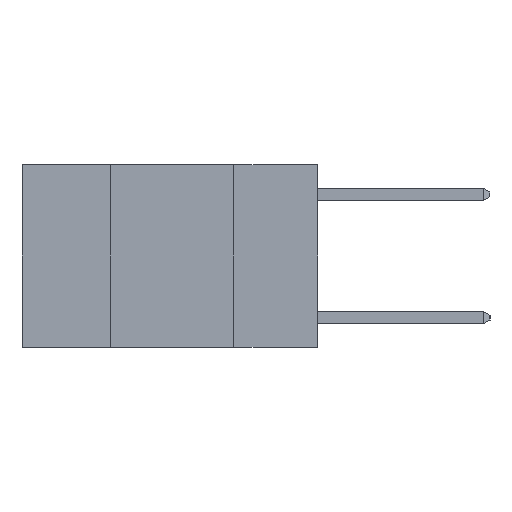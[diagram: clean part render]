
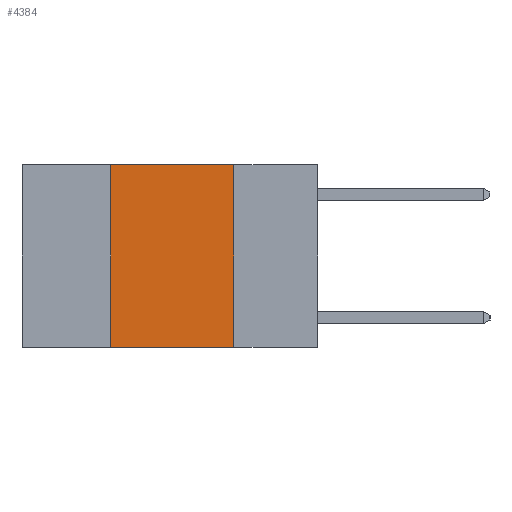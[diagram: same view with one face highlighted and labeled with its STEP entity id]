
A CAD part, left-side view. The second image highlights one B-rep face of the part: STEP entity #4384.
In plain terms, the highlighted planar face has unit normal (-1, 0, 0).
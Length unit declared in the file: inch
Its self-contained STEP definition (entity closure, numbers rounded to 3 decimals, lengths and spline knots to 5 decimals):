
#408 = CARTESIAN_POINT ( 'NONE',  ( 0., 0.17, 0. ) ) ;
#870 = FACE_OUTER_BOUND ( 'NONE', #2531, .T. ) ;
#1469 = CARTESIAN_POINT ( 'NONE',  ( 0., 0.42, -0.37 ) ) ;
#1685 = VERTEX_POINT ( 'NONE', #2592 ) ;
#1968 = VERTEX_POINT ( 'NONE', #1469 ) ;
#2078 = CARTESIAN_POINT ( 'NONE',  ( 0., 0.17, 0. ) ) ;
#2221 = VECTOR ( 'NONE', #9782, 39.37008 ) ;
#2294 = VECTOR ( 'NONE', #6770, 39.37008 ) ;
#2531 = EDGE_LOOP ( 'NONE', ( #7770, #8087, #8686, #8904 ) ) ;
#2549 = LINE ( 'NONE', #9661, #2294 ) ;
#2592 = CARTESIAN_POINT ( 'NONE',  ( 0., 0.17, -0.37 ) ) ;
#2952 = CARTESIAN_POINT ( 'NONE',  ( 0., 0.6, 0. ) ) ;
#3485 = EDGE_CURVE ( 'NONE', #1968, #1685, #4253, .T. ) ;
#3518 = AXIS2_PLACEMENT_3D ( 'NONE', #4812, #4655, #4646 ) ;
#4253 = LINE ( 'NONE', #9540, #8129 ) ;
#4369 = LINE ( 'NONE', #2078, #2221 ) ;
#4384 = ADVANCED_FACE ( 'NONE', ( #870 ), #4664, .F. ) ;
#4646 = DIRECTION ( 'NONE',  ( 0., 0., -1. ) ) ;
#4655 = DIRECTION ( 'NONE',  ( 1., 0., 0. ) ) ;
#4664 = PLANE ( 'NONE',  #3518 ) ;
#4812 = CARTESIAN_POINT ( 'NONE',  ( 0., 0.6, 0. ) ) ;
#4862 = VECTOR ( 'NONE', #5391, 39.37008 ) ;
#5391 = DIRECTION ( 'NONE',  ( 0., -1., 0. ) ) ;
#5661 = CARTESIAN_POINT ( 'NONE',  ( 0., 0.42, 0. ) ) ;
#6770 = DIRECTION ( 'NONE',  ( 0., 0., 1. ) ) ;
#6971 = LINE ( 'NONE', #2952, #4862 ) ;
#7257 = EDGE_CURVE ( 'NONE', #7994, #1685, #4369, .T. ) ;
#7770 = ORIENTED_EDGE ( 'NONE', *, *, #7257, .F. ) ;
#7994 = VERTEX_POINT ( 'NONE', #408 ) ;
#8087 = ORIENTED_EDGE ( 'NONE', *, *, #8237, .F. ) ;
#8129 = VECTOR ( 'NONE', #9504, 39.37008 ) ;
#8237 = EDGE_CURVE ( 'NONE', #8413, #7994, #6971, .T. ) ;
#8413 = VERTEX_POINT ( 'NONE', #5661 ) ;
#8686 = ORIENTED_EDGE ( 'NONE', *, *, #9612, .F. ) ;
#8904 = ORIENTED_EDGE ( 'NONE', *, *, #3485, .T. ) ;
#9504 = DIRECTION ( 'NONE',  ( 0., -1., 0. ) ) ;
#9540 = CARTESIAN_POINT ( 'NONE',  ( 0., 0.6, -0.37 ) ) ;
#9612 = EDGE_CURVE ( 'NONE', #1968, #8413, #2549, .T. ) ;
#9661 = CARTESIAN_POINT ( 'NONE',  ( 0., 0.42, 0. ) ) ;
#9782 = DIRECTION ( 'NONE',  ( 0., 0., -1. ) ) ;
